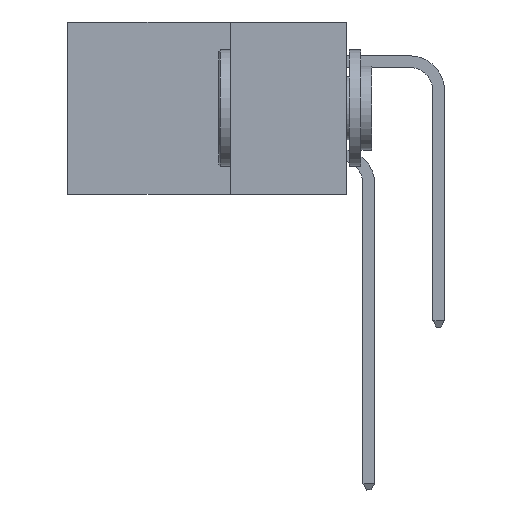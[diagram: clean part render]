
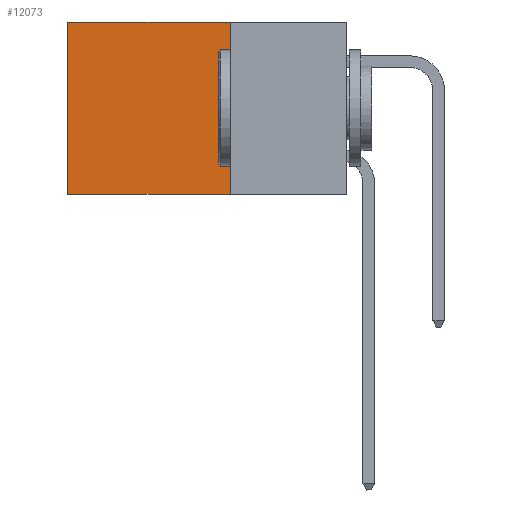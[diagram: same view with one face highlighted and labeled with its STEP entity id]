
A CAD part, left-side view. The second image highlights one B-rep face of the part: STEP entity #12073.
In plain terms, the highlighted planar face has unit normal (-1, 0, 0).
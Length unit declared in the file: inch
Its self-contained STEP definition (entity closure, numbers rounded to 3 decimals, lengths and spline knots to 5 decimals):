
#293 = EDGE_CURVE ( 'NONE', #1081, #3354, #12077, .T. ) ;
#351 = CARTESIAN_POINT ( 'NONE',  ( 0.2875, 0.25, 0. ) ) ;
#658 = EDGE_CURVE ( 'NONE', #3066, #2315, #1975, .T. ) ;
#1073 = AXIS2_PLACEMENT_3D ( 'NONE', #9039, #8237, #5215 ) ;
#1081 = VERTEX_POINT ( 'NONE', #9812 ) ;
#1507 = PLANE ( 'NONE',  #1073 ) ;
#1594 = ORIENTED_EDGE ( 'NONE', *, *, #658, .T. ) ;
#1975 = LINE ( 'NONE', #3342, #4991 ) ;
#2063 = LINE ( 'NONE', #11836, #2352 ) ;
#2315 = VERTEX_POINT ( 'NONE', #9047 ) ;
#2352 = VECTOR ( 'NONE', #8067, 39.37008 ) ;
#3021 = EDGE_CURVE ( 'NONE', #2315, #3354, #2063, .T. ) ;
#3066 = VERTEX_POINT ( 'NONE', #351 ) ;
#3342 = CARTESIAN_POINT ( 'NONE',  ( 0.2875, 0.25, 0. ) ) ;
#3354 = VERTEX_POINT ( 'NONE', #8739 ) ;
#3960 = EDGE_CURVE ( 'NONE', #3066, #1081, #7640, .T. ) ;
#4537 = ORIENTED_EDGE ( 'NONE', *, *, #293, .F. ) ;
#4754 = DIRECTION ( 'NONE',  ( 0., 1., 0. ) ) ;
#4991 = VECTOR ( 'NONE', #10100, 39.37008 ) ;
#5215 = DIRECTION ( 'NONE',  ( 0., 0., -1. ) ) ;
#5330 = ORIENTED_EDGE ( 'NONE', *, *, #3960, .F. ) ;
#5411 = CARTESIAN_POINT ( 'NONE',  ( 0.2875, 0.25, -0.37 ) ) ;
#5696 = VECTOR ( 'NONE', #6594, 39.37008 ) ;
#6594 = DIRECTION ( 'NONE',  ( 0., 0., -1. ) ) ;
#7394 = VECTOR ( 'NONE', #4754, 39.37008 ) ;
#7640 = LINE ( 'NONE', #10411, #5696 ) ;
#8067 = DIRECTION ( 'NONE',  ( 0., 0., -1. ) ) ;
#8237 = DIRECTION ( 'NONE',  ( 1., 0., 0. ) ) ;
#8739 = CARTESIAN_POINT ( 'NONE',  ( 0.2875, 0.6, -0.37 ) ) ;
#8894 = EDGE_LOOP ( 'NONE', ( #11367, #4537, #5330, #1594 ) ) ;
#9039 = CARTESIAN_POINT ( 'NONE',  ( 0.2875, 0.25, 0. ) ) ;
#9047 = CARTESIAN_POINT ( 'NONE',  ( 0.2875, 0.6, 0. ) ) ;
#9812 = CARTESIAN_POINT ( 'NONE',  ( 0.2875, 0.25, -0.37 ) ) ;
#10100 = DIRECTION ( 'NONE',  ( 0., 1., 0. ) ) ;
#10411 = CARTESIAN_POINT ( 'NONE',  ( 0.2875, 0.25, 0. ) ) ;
#11367 = ORIENTED_EDGE ( 'NONE', *, *, #3021, .T. ) ;
#11836 = CARTESIAN_POINT ( 'NONE',  ( 0.2875, 0.6, 0. ) ) ;
#12073 = ADVANCED_FACE ( 'NONE', ( #12463 ), #1507, .F. ) ;
#12077 = LINE ( 'NONE', #5411, #7394 ) ;
#12463 = FACE_OUTER_BOUND ( 'NONE', #8894, .T. ) ;
